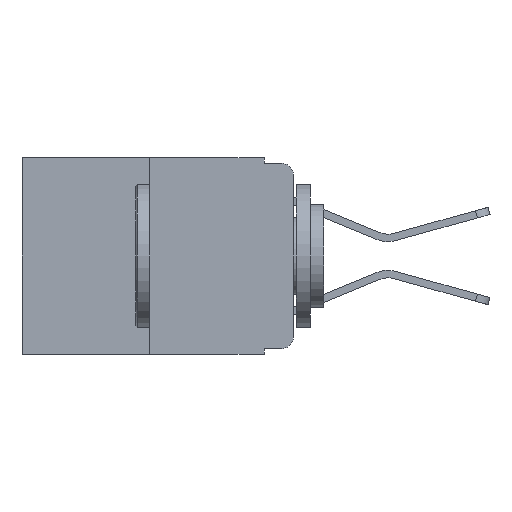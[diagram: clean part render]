
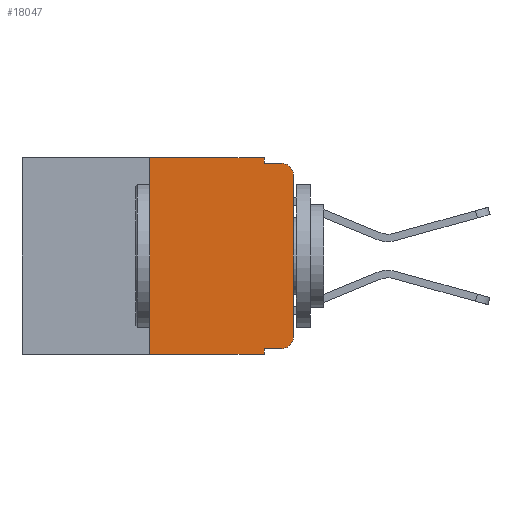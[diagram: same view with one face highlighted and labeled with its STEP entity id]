
A CAD part, left-side view. The second image highlights one B-rep face of the part: STEP entity #18047.
In plain terms, the highlighted planar face has unit normal (-1, 0, 0).
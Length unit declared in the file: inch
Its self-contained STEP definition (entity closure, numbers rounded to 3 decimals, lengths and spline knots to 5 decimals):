
#78 = VERTEX_POINT ( 'NONE', #4522 ) ;
#188 = DIRECTION ( 'NONE',  ( 0., 0., -1. ) ) ;
#260 = DIRECTION ( 'NONE',  ( 0., 0., -1. ) ) ;
#509 = VECTOR ( 'NONE', #9654, 39.37008 ) ;
#655 = EDGE_CURVE ( 'NONE', #15195, #17175, #14133, .T. ) ;
#721 = ORIENTED_EDGE ( 'NONE', *, *, #18034, .F. ) ;
#1051 = CARTESIAN_POINT ( 'NONE',  ( 0., 0.051, -0.01 ) ) ;
#1275 = ORIENTED_EDGE ( 'NONE', *, *, #15858, .F. ) ;
#1408 = CARTESIAN_POINT ( 'NONE',  ( 0., 0.02, -0.313 ) ) ;
#2064 = CARTESIAN_POINT ( 'NONE',  ( 0., 0.051, 0. ) ) ;
#3259 = DIRECTION ( 'NONE',  ( 0., 0., -1. ) ) ;
#3866 = EDGE_CURVE ( 'NONE', #18867, #78, #15843, .T. ) ;
#4092 = CARTESIAN_POINT ( 'NONE',  ( 0., 0., -0.03 ) ) ;
#4522 = CARTESIAN_POINT ( 'NONE',  ( 0., 0.25, 0. ) ) ;
#4685 = VECTOR ( 'NONE', #10958, 39.37008 ) ;
#4733 = VERTEX_POINT ( 'NONE', #11175 ) ;
#5282 = VECTOR ( 'NONE', #11409, 39.37008 ) ;
#5458 = CARTESIAN_POINT ( 'NONE',  ( 0., 0.02, -0.01 ) ) ;
#6530 = VERTEX_POINT ( 'NONE', #10434 ) ;
#6532 = VECTOR ( 'NONE', #7408, 39.37008 ) ;
#6676 = CARTESIAN_POINT ( 'NONE',  ( 0., 0.02, -0.333 ) ) ;
#6972 = ORIENTED_EDGE ( 'NONE', *, *, #12546, .T. ) ;
#7371 = VECTOR ( 'NONE', #13896, 39.37008 ) ;
#7408 = DIRECTION ( 'NONE',  ( 0., 0., 1. ) ) ;
#7813 = ORIENTED_EDGE ( 'NONE', *, *, #20703, .T. ) ;
#7978 = CARTESIAN_POINT ( 'NONE',  ( 0., 0.02, -0.03 ) ) ;
#8724 = LINE ( 'NONE', #12648, #17436 ) ;
#8864 = VECTOR ( 'NONE', #13246, 39.37008 ) ;
#8900 = LINE ( 'NONE', #21280, #4685 ) ;
#9654 = DIRECTION ( 'NONE',  ( 0., 0., 1. ) ) ;
#9767 = DIRECTION ( 'NONE',  ( 0., 0., -1. ) ) ;
#9817 = CARTESIAN_POINT ( 'NONE',  ( 0., 0.473, 0. ) ) ;
#10150 = CIRCLE ( 'NONE', #20204, 0.02 ) ;
#10434 = CARTESIAN_POINT ( 'NONE',  ( 0., 0., -0.313 ) ) ;
#10671 = LINE ( 'NONE', #16639, #509 ) ;
#10923 = LINE ( 'NONE', #2064, #21177 ) ;
#10958 = DIRECTION ( 'NONE',  ( 0., -1., 0. ) ) ;
#10991 = DIRECTION ( 'NONE',  ( 1., 0., 0. ) ) ;
#11175 = CARTESIAN_POINT ( 'NONE',  ( 0., 0.051, 0. ) ) ;
#11409 = DIRECTION ( 'NONE',  ( 0., -1., 0. ) ) ;
#11525 = CARTESIAN_POINT ( 'NONE',  ( 0., 0.051, -0.333 ) ) ;
#11651 = CARTESIAN_POINT ( 'NONE',  ( 0., 0.051, -0.333 ) ) ;
#11659 = VERTEX_POINT ( 'NONE', #5458 ) ;
#11719 = CARTESIAN_POINT ( 'NONE',  ( 0., 0.25, -0.343 ) ) ;
#11809 = VERTEX_POINT ( 'NONE', #4092 ) ;
#12151 = CARTESIAN_POINT ( 'NONE',  ( 0., 0.051, -0.01 ) ) ;
#12546 = EDGE_CURVE ( 'NONE', #6530, #11809, #10671, .T. ) ;
#12648 = CARTESIAN_POINT ( 'NONE',  ( 0., 0.051, 0. ) ) ;
#12785 = EDGE_CURVE ( 'NONE', #17175, #6530, #10150, .T. ) ;
#12843 = FACE_OUTER_BOUND ( 'NONE', #22173, .T. ) ;
#13246 = DIRECTION ( 'NONE',  ( 0., -1., 0. ) ) ;
#13844 = EDGE_CURVE ( 'NONE', #15195, #16021, #10923, .T. ) ;
#13896 = DIRECTION ( 'NONE',  ( 0., -1., 0. ) ) ;
#13906 = DIRECTION ( 'NONE',  ( -1., 0., 0. ) ) ;
#14131 = ORIENTED_EDGE ( 'NONE', *, *, #12785, .T. ) ;
#14133 = LINE ( 'NONE', #11651, #5282 ) ;
#14320 = AXIS2_PLACEMENT_3D ( 'NONE', #17859, #10991, #188 ) ;
#15195 = VERTEX_POINT ( 'NONE', #11525 ) ;
#15843 = LINE ( 'NONE', #16632, #6532 ) ;
#15858 = EDGE_CURVE ( 'NONE', #78, #4733, #18121, .T. ) ;
#16012 = ORIENTED_EDGE ( 'NONE', *, *, #3866, .F. ) ;
#16021 = VERTEX_POINT ( 'NONE', #20627 ) ;
#16117 = LINE ( 'NONE', #12151, #7371 ) ;
#16632 = CARTESIAN_POINT ( 'NONE',  ( 0., 0.25, 0. ) ) ;
#16639 = CARTESIAN_POINT ( 'NONE',  ( 0., 0., 0. ) ) ;
#17175 = VERTEX_POINT ( 'NONE', #6676 ) ;
#17436 = VECTOR ( 'NONE', #21238, 39.37008 ) ;
#17606 = EDGE_CURVE ( 'NONE', #11809, #11659, #17998, .T. ) ;
#17642 = ORIENTED_EDGE ( 'NONE', *, *, #13844, .F. ) ;
#17859 = CARTESIAN_POINT ( 'NONE',  ( 0., 0.473, 0. ) ) ;
#17998 = CIRCLE ( 'NONE', #19499, 0.02 ) ;
#18034 = EDGE_CURVE ( 'NONE', #4733, #18266, #8724, .T. ) ;
#18047 = ADVANCED_FACE ( 'NONE', ( #12843 ), #21309, .F. ) ;
#18121 = LINE ( 'NONE', #9817, #8864 ) ;
#18266 = VERTEX_POINT ( 'NONE', #1051 ) ;
#18867 = VERTEX_POINT ( 'NONE', #11719 ) ;
#18992 = ORIENTED_EDGE ( 'NONE', *, *, #22617, .F. ) ;
#19499 = AXIS2_PLACEMENT_3D ( 'NONE', #7978, #20143, #9767 ) ;
#20143 = DIRECTION ( 'NONE',  ( -1., 0., 0. ) ) ;
#20204 = AXIS2_PLACEMENT_3D ( 'NONE', #1408, #13906, #3259 ) ;
#20627 = CARTESIAN_POINT ( 'NONE',  ( 0., 0.051, -0.343 ) ) ;
#20703 = EDGE_CURVE ( 'NONE', #18867, #16021, #8900, .T. ) ;
#21177 = VECTOR ( 'NONE', #260, 39.37008 ) ;
#21238 = DIRECTION ( 'NONE',  ( 0., 0., -1. ) ) ;
#21280 = CARTESIAN_POINT ( 'NONE',  ( 0., 0.473, -0.343 ) ) ;
#21309 = PLANE ( 'NONE',  #14320 ) ;
#22173 = EDGE_LOOP ( 'NONE', ( #6972, #22457, #18992, #721, #1275, #16012, #7813, #17642, #22198, #14131 ) ) ;
#22198 = ORIENTED_EDGE ( 'NONE', *, *, #655, .T. ) ;
#22457 = ORIENTED_EDGE ( 'NONE', *, *, #17606, .T. ) ;
#22617 = EDGE_CURVE ( 'NONE', #18266, #11659, #16117, .T. ) ;
